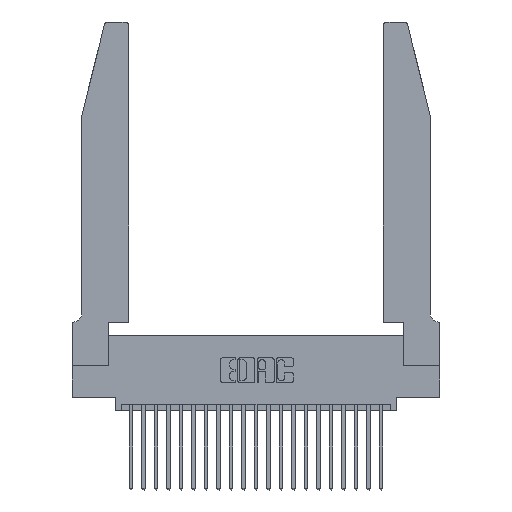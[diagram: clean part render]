
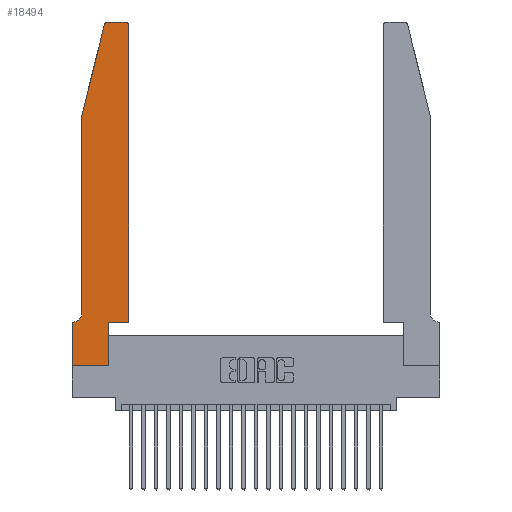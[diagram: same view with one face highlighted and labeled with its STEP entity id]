
A CAD part, top view. The second image highlights one B-rep face of the part: STEP entity #18494.
In plain terms, the highlighted planar face has unit normal (0, 0, 1).
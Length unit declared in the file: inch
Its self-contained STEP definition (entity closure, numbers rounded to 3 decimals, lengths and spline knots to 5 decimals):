
#133 = VERTEX_POINT ( 'NONE', #2349 ) ;
#348 = LINE ( 'NONE', #22216, #20434 ) ;
#709 = DIRECTION ( 'NONE',  ( 1., 0., 0. ) ) ;
#756 = ORIENTED_EDGE ( 'NONE', *, *, #12238, .T. ) ;
#842 = LINE ( 'NONE', #22086, #19752 ) ;
#850 = CARTESIAN_POINT ( 'NONE',  ( 0.25487, 2.72718, 0.37 ) ) ;
#955 = CARTESIAN_POINT ( 'NONE',  ( 0.0755, 2., 0.37 ) ) ;
#1082 = VERTEX_POINT ( 'NONE', #22209 ) ;
#1227 = ORIENTED_EDGE ( 'NONE', *, *, #15536, .T. ) ;
#1315 = LINE ( 'NONE', #16669, #19627 ) ;
#1459 = LINE ( 'NONE', #955, #15437 ) ;
#1544 = VECTOR ( 'NONE', #18645, 39.37008 ) ;
#2349 = CARTESIAN_POINT ( 'NONE',  ( 0., 0., 0.37 ) ) ;
#2689 = ORIENTED_EDGE ( 'NONE', *, *, #14406, .T. ) ;
#2745 = VERTEX_POINT ( 'NONE', #16753 ) ;
#2886 = CIRCLE ( 'NONE', #10477, 0.03 ) ;
#2898 = DIRECTION ( 'NONE',  ( -0.239, -0.971, 0. ) ) ;
#3140 = CARTESIAN_POINT ( 'NONE',  ( 0.0055, 0.35, 0.37 ) ) ;
#3552 = LINE ( 'NONE', #21950, #22262 ) ;
#3795 = DIRECTION ( 'NONE',  ( 0., 0., -1. ) ) ;
#4231 = CARTESIAN_POINT ( 'NONE',  ( 0.4205, 2.75, 0.37 ) ) ;
#4233 = ORIENTED_EDGE ( 'NONE', *, *, #7901, .T. ) ;
#4318 = CARTESIAN_POINT ( 'NONE',  ( 0.2865, 0., 0.37 ) ) ;
#5275 = DIRECTION ( 'NONE',  ( 0., 1., 0. ) ) ;
#5711 = LINE ( 'NONE', #20555, #14643 ) ;
#7085 = EDGE_CURVE ( 'NONE', #2745, #11939, #2886, .T. ) ;
#7160 = AXIS2_PLACEMENT_3D ( 'NONE', #15166, #3795, #17053 ) ;
#7234 = CIRCLE ( 'NONE', #18038, 0.03 ) ;
#7300 = ORIENTED_EDGE ( 'NONE', *, *, #7085, .T. ) ;
#7318 = CARTESIAN_POINT ( 'NONE',  ( 0.4505, 0.35, 0.37 ) ) ;
#7395 = DIRECTION ( 'NONE',  ( 1., 0., 0. ) ) ;
#7746 = EDGE_CURVE ( 'NONE', #1082, #10725, #22447, .T. ) ;
#7901 = EDGE_CURVE ( 'NONE', #10725, #2745, #20220, .T. ) ;
#8070 = EDGE_LOOP ( 'NONE', ( #19740, #23664, #17425, #756, #16961, #1227, #16332, #2689, #15303, #23672, #4233, #7300 ) ) ;
#8422 = CARTESIAN_POINT ( 'NONE',  ( 0.4205, 2.72, 0.37 ) ) ;
#8481 = PLANE ( 'NONE',  #18689 ) ;
#8916 = DIRECTION ( 'NONE',  ( 0., -1., 0. ) ) ;
#9004 = EDGE_CURVE ( 'NONE', #15617, #133, #1315, .T. ) ;
#9781 = VERTEX_POINT ( 'NONE', #13571 ) ;
#10140 = EDGE_CURVE ( 'NONE', #19436, #16660, #7234, .T. ) ;
#10330 = VECTOR ( 'NONE', #13658, 39.37008 ) ;
#10361 = DIRECTION ( 'NONE',  ( 1., 0., 0. ) ) ;
#10412 = DIRECTION ( 'NONE',  ( 0., 0., 1. ) ) ;
#10474 = EDGE_CURVE ( 'NONE', #11939, #19436, #5711, .T. ) ;
#10477 = AXIS2_PLACEMENT_3D ( 'NONE', #8422, #21430, #10361 ) ;
#10725 = VERTEX_POINT ( 'NONE', #17522 ) ;
#11761 = CARTESIAN_POINT ( 'NONE',  ( 0.4505, 0.35, 0.37 ) ) ;
#11939 = VERTEX_POINT ( 'NONE', #4231 ) ;
#12098 = EDGE_CURVE ( 'NONE', #16660, #20681, #1459, .T. ) ;
#12197 = DIRECTION ( 'NONE',  ( 0., 0., 1. ) ) ;
#12238 = EDGE_CURVE ( 'NONE', #20681, #9781, #3552, .T. ) ;
#12729 = VECTOR ( 'NONE', #7395, 39.37008 ) ;
#12935 = LINE ( 'NONE', #16709, #1544 ) ;
#13571 = CARTESIAN_POINT ( 'NONE',  ( 0.0755, 0.42, 0.37 ) ) ;
#13658 = DIRECTION ( 'NONE',  ( 0., 1., 0. ) ) ;
#14406 = EDGE_CURVE ( 'NONE', #133, #21549, #348, .T. ) ;
#14643 = VECTOR ( 'NONE', #22330, 39.37008 ) ;
#14883 = DIRECTION ( 'NONE',  ( 1., 0., 0. ) ) ;
#15166 = CARTESIAN_POINT ( 'NONE',  ( 0.0055, 0.42, 0.37 ) ) ;
#15303 = ORIENTED_EDGE ( 'NONE', *, *, #20563, .T. ) ;
#15437 = VECTOR ( 'NONE', #2898, 39.37008 ) ;
#15536 = EDGE_CURVE ( 'NONE', #20504, #15617, #12935, .T. ) ;
#15617 = VERTEX_POINT ( 'NONE', #24194 ) ;
#15728 = CARTESIAN_POINT ( 'NONE',  ( 0.0755, 2., 0.37 ) ) ;
#16332 = ORIENTED_EDGE ( 'NONE', *, *, #9004, .T. ) ;
#16425 = EDGE_CURVE ( 'NONE', #9781, #20504, #19526, .T. ) ;
#16660 = VERTEX_POINT ( 'NONE', #850 ) ;
#16669 = CARTESIAN_POINT ( 'NONE',  ( 0., 0., 0.37 ) ) ;
#16709 = CARTESIAN_POINT ( 'NONE',  ( 0.0755, 0.35, 0.37 ) ) ;
#16753 = CARTESIAN_POINT ( 'NONE',  ( 0.4505, 2.72, 0.37 ) ) ;
#16961 = ORIENTED_EDGE ( 'NONE', *, *, #16425, .T. ) ;
#17053 = DIRECTION ( 'NONE',  ( -1., 0., 0. ) ) ;
#17250 = CARTESIAN_POINT ( 'NONE',  ( 0.284, 2.75, 0.37 ) ) ;
#17425 = ORIENTED_EDGE ( 'NONE', *, *, #12098, .T. ) ;
#17429 = FACE_OUTER_BOUND ( 'NONE', #8070, .T. ) ;
#17522 = CARTESIAN_POINT ( 'NONE',  ( 0.4505, 0.35, 0.37 ) ) ;
#18038 = AXIS2_PLACEMENT_3D ( 'NONE', #23131, #12197, #709 ) ;
#18494 = ADVANCED_FACE ( 'NONE', ( #17429 ), #8481, .T. ) ;
#18645 = DIRECTION ( 'NONE',  ( -1., 0., 0. ) ) ;
#18689 = AXIS2_PLACEMENT_3D ( 'NONE', #21476, #10412, #23272 ) ;
#19436 = VERTEX_POINT ( 'NONE', #17250 ) ;
#19526 = CIRCLE ( 'NONE', #7160, 0.07 ) ;
#19627 = VECTOR ( 'NONE', #22132, 39.37008 ) ;
#19740 = ORIENTED_EDGE ( 'NONE', *, *, #10474, .T. ) ;
#19752 = VECTOR ( 'NONE', #5275, 39.37008 ) ;
#20220 = LINE ( 'NONE', #11761, #10330 ) ;
#20434 = VECTOR ( 'NONE', #14883, 39.37008 ) ;
#20504 = VERTEX_POINT ( 'NONE', #3140 ) ;
#20555 = CARTESIAN_POINT ( 'NONE',  ( 0.2605, 2.75, 0.37 ) ) ;
#20563 = EDGE_CURVE ( 'NONE', #21549, #1082, #842, .T. ) ;
#20681 = VERTEX_POINT ( 'NONE', #15728 ) ;
#21430 = DIRECTION ( 'NONE',  ( 0., 0., 1. ) ) ;
#21476 = CARTESIAN_POINT ( 'NONE',  ( 0., 0.35, 0.37 ) ) ;
#21549 = VERTEX_POINT ( 'NONE', #4318 ) ;
#21950 = CARTESIAN_POINT ( 'NONE',  ( 0.0755, 2., 0.37 ) ) ;
#22086 = CARTESIAN_POINT ( 'NONE',  ( 0.2865, 0.35, 0.37 ) ) ;
#22132 = DIRECTION ( 'NONE',  ( 0., -1., 0. ) ) ;
#22209 = CARTESIAN_POINT ( 'NONE',  ( 0.2865, 0.35, 0.37 ) ) ;
#22216 = CARTESIAN_POINT ( 'NONE',  ( 0., 0., 0.37 ) ) ;
#22262 = VECTOR ( 'NONE', #8916, 39.37008 ) ;
#22330 = DIRECTION ( 'NONE',  ( -1., 0., 0. ) ) ;
#22447 = LINE ( 'NONE', #7318, #12729 ) ;
#23131 = CARTESIAN_POINT ( 'NONE',  ( 0.284, 2.72, 0.37 ) ) ;
#23272 = DIRECTION ( 'NONE',  ( 1., 0., 0. ) ) ;
#23664 = ORIENTED_EDGE ( 'NONE', *, *, #10140, .T. ) ;
#23672 = ORIENTED_EDGE ( 'NONE', *, *, #7746, .T. ) ;
#24194 = CARTESIAN_POINT ( 'NONE',  ( 0., 0.35, 0.37 ) ) ;
